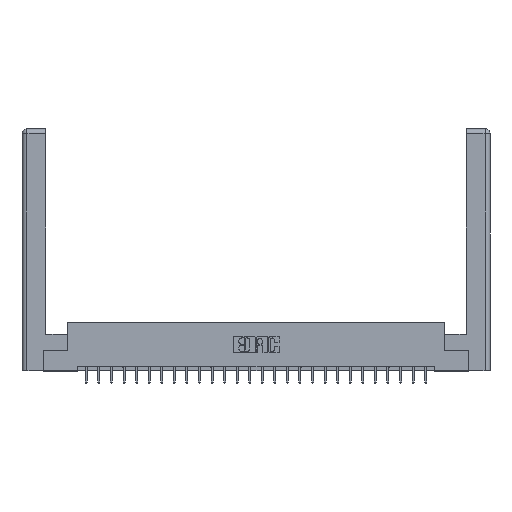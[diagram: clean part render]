
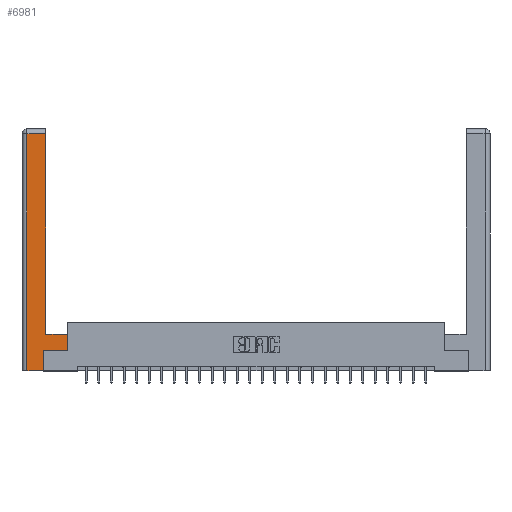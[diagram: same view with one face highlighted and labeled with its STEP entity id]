
A CAD part, top view. The second image highlights one B-rep face of the part: STEP entity #6981.
In plain terms, the highlighted planar face has unit normal (0, 0, 1).
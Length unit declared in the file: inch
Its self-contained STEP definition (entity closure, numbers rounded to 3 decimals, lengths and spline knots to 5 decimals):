
#1212 = FACE_OUTER_BOUND ( 'NONE', #17320, .T. ) ;
#1568 = VECTOR ( 'NONE', #19361, 39.37008 ) ;
#1783 = ORIENTED_EDGE ( 'NONE', *, *, #13890, .T. ) ;
#1814 = VECTOR ( 'NONE', #10171, 39.37008 ) ;
#2831 = VERTEX_POINT ( 'NONE', #15887 ) ;
#3017 = CARTESIAN_POINT ( 'NONE',  ( 0.265, 0.245, 0. ) ) ;
#4222 = CARTESIAN_POINT ( 'NONE',  ( 0.0615, 2.94, 0. ) ) ;
#4589 = CARTESIAN_POINT ( 'NONE',  ( 0.295, 0.45, 0. ) ) ;
#5221 = EDGE_CURVE ( 'NONE', #19627, #17147, #13910, .T. ) ;
#5367 = EDGE_CURVE ( 'NONE', #2831, #10408, #17994, .T. ) ;
#5516 = LINE ( 'NONE', #19053, #14323 ) ;
#6301 = CARTESIAN_POINT ( 'NONE',  ( 0.265, 0., 0. ) ) ;
#6720 = EDGE_CURVE ( 'NONE', #12507, #25550, #19212, .T. ) ;
#6926 = LINE ( 'NONE', #14919, #1568 ) ;
#6951 = DIRECTION ( 'NONE',  ( 1., 0., 0. ) ) ;
#6981 = ADVANCED_FACE ( 'NONE', ( #1212 ), #8326, .F. ) ;
#7167 = LINE ( 'NONE', #22221, #1814 ) ;
#7263 = VECTOR ( 'NONE', #15376, 39.37008 ) ;
#7533 = CARTESIAN_POINT ( 'NONE',  ( 0.0615, 0., 0. ) ) ;
#8326 = PLANE ( 'NONE',  #9313 ) ;
#8414 = CARTESIAN_POINT ( 'NONE',  ( 0., 0., 0. ) ) ;
#8562 = VECTOR ( 'NONE', #19204, 39.37008 ) ;
#9313 = AXIS2_PLACEMENT_3D ( 'NONE', #8414, #22485, #16329 ) ;
#9690 = VECTOR ( 'NONE', #23177, 39.37008 ) ;
#10171 = DIRECTION ( 'NONE',  ( 0., -1., 0. ) ) ;
#10408 = VERTEX_POINT ( 'NONE', #16845 ) ;
#10650 = ORIENTED_EDGE ( 'NONE', *, *, #6720, .T. ) ;
#10664 = VECTOR ( 'NONE', #22496, 39.37008 ) ;
#11814 = VERTEX_POINT ( 'NONE', #22955 ) ;
#12232 = ORIENTED_EDGE ( 'NONE', *, *, #22599, .T. ) ;
#12507 = VERTEX_POINT ( 'NONE', #7533 ) ;
#12986 = LINE ( 'NONE', #4222, #15829 ) ;
#13700 = CARTESIAN_POINT ( 'NONE',  ( 0.565, 0.45, 0. ) ) ;
#13890 = EDGE_CURVE ( 'NONE', #25550, #11814, #23020, .T. ) ;
#13910 = LINE ( 'NONE', #21167, #8562 ) ;
#13958 = CARTESIAN_POINT ( 'NONE',  ( 0.295, 2.94, 0. ) ) ;
#14323 = VECTOR ( 'NONE', #6951, 39.37008 ) ;
#14645 = EDGE_CURVE ( 'NONE', #19712, #12507, #7167, .T. ) ;
#14853 = CARTESIAN_POINT ( 'NONE',  ( 0.0615, 2.94, 0. ) ) ;
#14919 = CARTESIAN_POINT ( 'NONE',  ( 0.295, 0.45, 0. ) ) ;
#15376 = DIRECTION ( 'NONE',  ( 0., 1., 0. ) ) ;
#15829 = VECTOR ( 'NONE', #18323, 39.37008 ) ;
#15887 = CARTESIAN_POINT ( 'NONE',  ( 0.565, 0.245, 0. ) ) ;
#16090 = ORIENTED_EDGE ( 'NONE', *, *, #5367, .T. ) ;
#16329 = DIRECTION ( 'NONE',  ( -1., 0., 0. ) ) ;
#16845 = CARTESIAN_POINT ( 'NONE',  ( 0.565, 0.45, 0. ) ) ;
#17147 = VERTEX_POINT ( 'NONE', #13958 ) ;
#17320 = EDGE_LOOP ( 'NONE', ( #23131, #12232, #23964, #10650, #1783, #22878, #16090, #24073 ) ) ;
#17994 = LINE ( 'NONE', #13700, #7263 ) ;
#18323 = DIRECTION ( 'NONE',  ( -1., 0., 0. ) ) ;
#18861 = EDGE_CURVE ( 'NONE', #10408, #19627, #6926, .T. ) ;
#19053 = CARTESIAN_POINT ( 'NONE',  ( 0.565, 0.245, 0. ) ) ;
#19204 = DIRECTION ( 'NONE',  ( 0., 1., 0. ) ) ;
#19212 = LINE ( 'NONE', #6301, #10664 ) ;
#19361 = DIRECTION ( 'NONE',  ( -1., 0., 0. ) ) ;
#19627 = VERTEX_POINT ( 'NONE', #4589 ) ;
#19712 = VERTEX_POINT ( 'NONE', #14853 ) ;
#20133 = CARTESIAN_POINT ( 'NONE',  ( 0.265, 0., 0. ) ) ;
#20856 = EDGE_CURVE ( 'NONE', #11814, #2831, #5516, .T. ) ;
#21167 = CARTESIAN_POINT ( 'NONE',  ( 0.295, 3., 0. ) ) ;
#22221 = CARTESIAN_POINT ( 'NONE',  ( 0.0615, 0., 0. ) ) ;
#22485 = DIRECTION ( 'NONE',  ( 0., 0., -1. ) ) ;
#22496 = DIRECTION ( 'NONE',  ( 1., 0., 0. ) ) ;
#22599 = EDGE_CURVE ( 'NONE', #17147, #19712, #12986, .T. ) ;
#22878 = ORIENTED_EDGE ( 'NONE', *, *, #20856, .T. ) ;
#22955 = CARTESIAN_POINT ( 'NONE',  ( 0.265, 0.245, 0. ) ) ;
#23020 = LINE ( 'NONE', #3017, #9690 ) ;
#23131 = ORIENTED_EDGE ( 'NONE', *, *, #5221, .T. ) ;
#23177 = DIRECTION ( 'NONE',  ( 0., 1., 0. ) ) ;
#23964 = ORIENTED_EDGE ( 'NONE', *, *, #14645, .T. ) ;
#24073 = ORIENTED_EDGE ( 'NONE', *, *, #18861, .T. ) ;
#25550 = VERTEX_POINT ( 'NONE', #20133 ) ;
